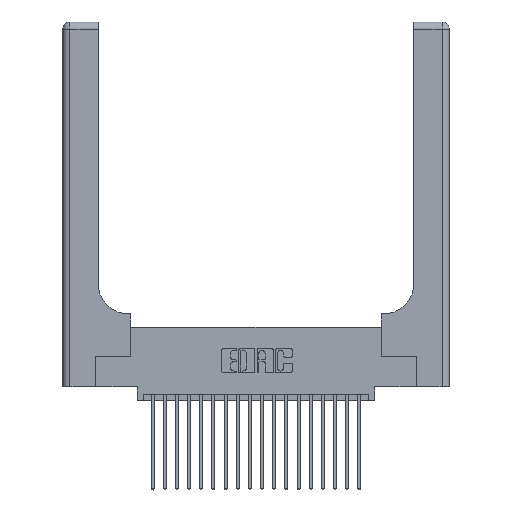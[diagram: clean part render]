
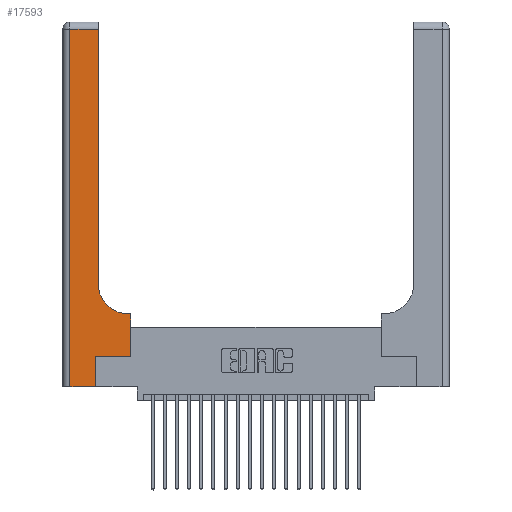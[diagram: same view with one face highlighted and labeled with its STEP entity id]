
A CAD part, top view. The second image highlights one B-rep face of the part: STEP entity #17593.
In plain terms, the highlighted planar face has unit normal (0, 0, 1).
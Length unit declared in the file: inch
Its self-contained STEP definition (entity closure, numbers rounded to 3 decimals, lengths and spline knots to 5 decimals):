
#75 = LINE ( 'NONE', #21586, #8351 ) ;
#98 = ORIENTED_EDGE ( 'NONE', *, *, #6678, .T. ) ;
#818 = DIRECTION ( 'NONE',  ( 1., 0., 0. ) ) ;
#1170 = VECTOR ( 'NONE', #15442, 39.37008 ) ;
#1415 = ORIENTED_EDGE ( 'NONE', *, *, #14732, .T. ) ;
#1420 = CARTESIAN_POINT ( 'NONE',  ( 0.5585, 0.6, 0.37 ) ) ;
#1455 = LINE ( 'NONE', #1628, #1170 ) ;
#1536 = EDGE_CURVE ( 'NONE', #14406, #13459, #14315, .T. ) ;
#1608 = LINE ( 'NONE', #20065, #22713 ) ;
#1628 = CARTESIAN_POINT ( 'NONE',  ( 0.269, 0.25, 0.37 ) ) ;
#1764 = CARTESIAN_POINT ( 'NONE',  ( 0.5415, 0.6, 0.37 ) ) ;
#2267 = VERTEX_POINT ( 'NONE', #1420 ) ;
#2788 = CARTESIAN_POINT ( 'NONE',  ( 0.2915, 0.85, 0.37 ) ) ;
#3044 = DIRECTION ( 'NONE',  ( 0., -1., 0. ) ) ;
#3070 = PLANE ( 'NONE',  #11178 ) ;
#3254 = CARTESIAN_POINT ( 'NONE',  ( 0.269, 0., 0.37 ) ) ;
#3559 = CARTESIAN_POINT ( 'NONE',  ( 0.06, 2.94, 0.37 ) ) ;
#3610 = ORIENTED_EDGE ( 'NONE', *, *, #8102, .T. ) ;
#3774 = DIRECTION ( 'NONE',  ( 0., 1., 0. ) ) ;
#4758 = LINE ( 'NONE', #18997, #14160 ) ;
#5297 = CARTESIAN_POINT ( 'NONE',  ( 0.2915, 2.94, 0.37 ) ) ;
#5495 = ORIENTED_EDGE ( 'NONE', *, *, #1536, .T. ) ;
#5791 = VERTEX_POINT ( 'NONE', #18679 ) ;
#5865 = ORIENTED_EDGE ( 'NONE', *, *, #20284, .T. ) ;
#5907 = EDGE_CURVE ( 'NONE', #22360, #14406, #4758, .T. ) ;
#5957 = DIRECTION ( 'NONE',  ( -1., 0., 0. ) ) ;
#6346 = EDGE_LOOP ( 'NONE', ( #15398, #19169, #5495, #3610, #98, #19928, #1415, #5865, #15520 ) ) ;
#6477 = EDGE_CURVE ( 'NONE', #5791, #17286, #1455, .T. ) ;
#6678 = EDGE_CURVE ( 'NONE', #6949, #5791, #14131, .T. ) ;
#6807 = VECTOR ( 'NONE', #3774, 39.37008 ) ;
#6949 = VERTEX_POINT ( 'NONE', #3254 ) ;
#7062 = EDGE_CURVE ( 'NONE', #8417, #10866, #12988, .T. ) ;
#7345 = LINE ( 'NONE', #16962, #19639 ) ;
#8073 = DIRECTION ( 'NONE',  ( 0., 1., 0. ) ) ;
#8102 = EDGE_CURVE ( 'NONE', #13459, #6949, #75, .T. ) ;
#8299 = CARTESIAN_POINT ( 'NONE',  ( 0., 3., 0.37 ) ) ;
#8351 = VECTOR ( 'NONE', #20049, 39.37008 ) ;
#8417 = VERTEX_POINT ( 'NONE', #1764 ) ;
#9253 = LINE ( 'NONE', #14023, #6807 ) ;
#9601 = DIRECTION ( 'NONE',  ( 0., 1., 0. ) ) ;
#10128 = CARTESIAN_POINT ( 'NONE',  ( 0.06, 3., 0.37 ) ) ;
#10790 = FACE_OUTER_BOUND ( 'NONE', #6346, .T. ) ;
#10831 = VECTOR ( 'NONE', #9601, 39.37008 ) ;
#10866 = VERTEX_POINT ( 'NONE', #2788 ) ;
#11067 = CARTESIAN_POINT ( 'NONE',  ( 0.06, 0., 0.37 ) ) ;
#11178 = AXIS2_PLACEMENT_3D ( 'NONE', #8299, #20532, #13389 ) ;
#11381 = CARTESIAN_POINT ( 'NONE',  ( 0.5415, 0.85, 0.37 ) ) ;
#12419 = VECTOR ( 'NONE', #3044, 39.37008 ) ;
#12480 = EDGE_CURVE ( 'NONE', #10866, #22360, #9253, .T. ) ;
#12988 = CIRCLE ( 'NONE', #20393, 0.25 ) ;
#13389 = DIRECTION ( 'NONE',  ( -1., 0., 0. ) ) ;
#13459 = VERTEX_POINT ( 'NONE', #11067 ) ;
#14023 = CARTESIAN_POINT ( 'NONE',  ( 0.2915, 3., 0.37 ) ) ;
#14131 = LINE ( 'NONE', #16406, #10831 ) ;
#14160 = VECTOR ( 'NONE', #22510, 39.37008 ) ;
#14315 = LINE ( 'NONE', #10128, #12419 ) ;
#14406 = VERTEX_POINT ( 'NONE', #3559 ) ;
#14732 = EDGE_CURVE ( 'NONE', #17286, #2267, #7345, .T. ) ;
#15398 = ORIENTED_EDGE ( 'NONE', *, *, #12480, .T. ) ;
#15442 = DIRECTION ( 'NONE',  ( 1., 0., 0. ) ) ;
#15520 = ORIENTED_EDGE ( 'NONE', *, *, #7062, .T. ) ;
#16406 = CARTESIAN_POINT ( 'NONE',  ( 0.269, 0., 0.37 ) ) ;
#16962 = CARTESIAN_POINT ( 'NONE',  ( 0.5585, 0.25, 0.37 ) ) ;
#16979 = CARTESIAN_POINT ( 'NONE',  ( 0.5585, 0.25, 0.37 ) ) ;
#17286 = VERTEX_POINT ( 'NONE', #16979 ) ;
#17593 = ADVANCED_FACE ( 'NONE', ( #10790 ), #3070, .F. ) ;
#18079 = DIRECTION ( 'NONE',  ( 0., 0., -1. ) ) ;
#18679 = CARTESIAN_POINT ( 'NONE',  ( 0.269, 0.25, 0.37 ) ) ;
#18997 = CARTESIAN_POINT ( 'NONE',  ( 0., 2.94, 0.37 ) ) ;
#19169 = ORIENTED_EDGE ( 'NONE', *, *, #5907, .T. ) ;
#19639 = VECTOR ( 'NONE', #8073, 39.37008 ) ;
#19928 = ORIENTED_EDGE ( 'NONE', *, *, #6477, .T. ) ;
#20049 = DIRECTION ( 'NONE',  ( 1., 0., 0. ) ) ;
#20065 = CARTESIAN_POINT ( 'NONE',  ( 0.2915, 0.6, 0.37 ) ) ;
#20284 = EDGE_CURVE ( 'NONE', #2267, #8417, #1608, .T. ) ;
#20393 = AXIS2_PLACEMENT_3D ( 'NONE', #11381, #18079, #818 ) ;
#20532 = DIRECTION ( 'NONE',  ( 0., 0., -1. ) ) ;
#21586 = CARTESIAN_POINT ( 'NONE',  ( 0., 0., 0.37 ) ) ;
#22360 = VERTEX_POINT ( 'NONE', #5297 ) ;
#22510 = DIRECTION ( 'NONE',  ( -1., 0., 0. ) ) ;
#22713 = VECTOR ( 'NONE', #5957, 39.37008 ) ;
